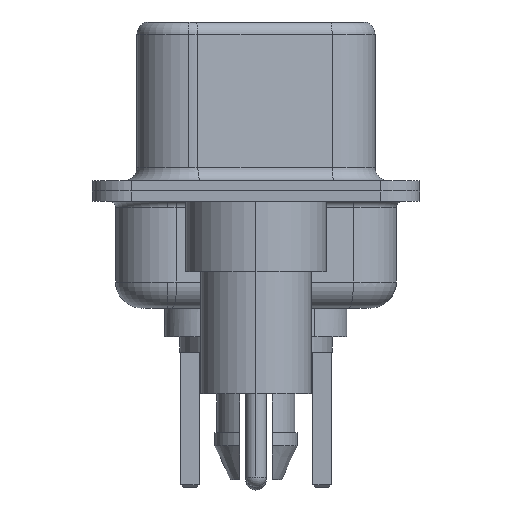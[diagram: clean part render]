
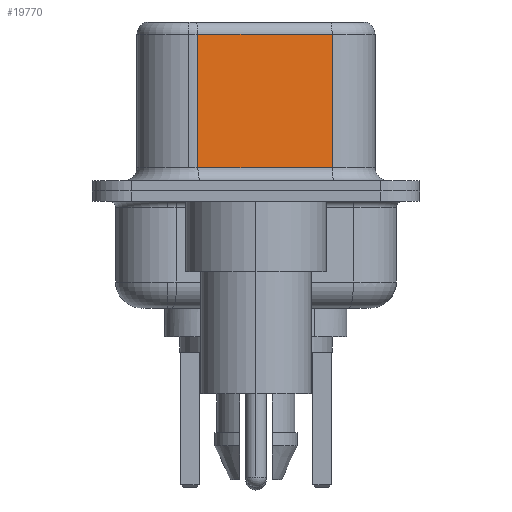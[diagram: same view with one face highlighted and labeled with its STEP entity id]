
A CAD part, left-side view. The second image highlights one B-rep face of the part: STEP entity #19770.
In plain terms, the highlighted planar face has unit normal (-0.985, -0.174, 0).
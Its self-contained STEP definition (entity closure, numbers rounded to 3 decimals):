
#413 = DIRECTION ( 'NONE',  ( -0.174, 0.985, 0. ) ) ;
#550 = LINE ( 'NONE', #19320, #12121 ) ;
#958 = EDGE_LOOP ( 'NONE', ( #11411, #16960, #17148, #9947 ) ) ;
#2748 = CARTESIAN_POINT ( 'NONE',  ( 4.565, -2.927, 6.02 ) ) ;
#3554 = EDGE_CURVE ( 'NONE', #14874, #12999, #9833, .T. ) ;
#4415 = PLANE ( 'NONE',  #17181 ) ;
#4439 = LINE ( 'NONE', #18417, #16595 ) ;
#6011 = DIRECTION ( 'NONE',  ( -0.174, 0.985, 0. ) ) ;
#6366 = FACE_OUTER_BOUND ( 'NONE', #958, .T. ) ;
#6947 = VECTOR ( 'NONE', #7154, 1000. ) ;
#7154 = DIRECTION ( 'NONE',  ( 0., 0., -1. ) ) ;
#7418 = CARTESIAN_POINT ( 'NONE',  ( 3.655, 2.233, 0.9 ) ) ;
#8909 = DIRECTION ( 'NONE',  ( 0., 0., -1. ) ) ;
#9833 = LINE ( 'NONE', #11067, #17757 ) ;
#9947 = ORIENTED_EDGE ( 'NONE', *, *, #3554, .T. ) ;
#10790 = CARTESIAN_POINT ( 'NONE',  ( 3.655, 2.233, 6.02 ) ) ;
#11067 = CARTESIAN_POINT ( 'NONE',  ( 4.565, -2.927, 0.9 ) ) ;
#11411 = ORIENTED_EDGE ( 'NONE', *, *, #14784, .F. ) ;
#11913 = CARTESIAN_POINT ( 'NONE',  ( 4.565, -2.927, 6.52 ) ) ;
#12121 = VECTOR ( 'NONE', #413, 1000. ) ;
#12999 = VERTEX_POINT ( 'NONE', #16021 ) ;
#13136 = DIRECTION ( 'NONE',  ( 0.174, -0.985, 0. ) ) ;
#14784 = EDGE_CURVE ( 'NONE', #19141, #12999, #14883, .T. ) ;
#14874 = VERTEX_POINT ( 'NONE', #7418 ) ;
#14883 = LINE ( 'NONE', #11913, #6947 ) ;
#15201 = EDGE_CURVE ( 'NONE', #19141, #16114, #550, .T. ) ;
#15424 = CARTESIAN_POINT ( 'NONE',  ( 4.565, -2.927, 6.52 ) ) ;
#15483 = EDGE_CURVE ( 'NONE', #16114, #14874, #4439, .T. ) ;
#15486 = DIRECTION ( 'NONE',  ( 0.985, 0.174, 0. ) ) ;
#16021 = CARTESIAN_POINT ( 'NONE',  ( 4.565, -2.927, 0.9 ) ) ;
#16114 = VERTEX_POINT ( 'NONE', #10790 ) ;
#16595 = VECTOR ( 'NONE', #8909, 1000. ) ;
#16960 = ORIENTED_EDGE ( 'NONE', *, *, #15201, .T. ) ;
#17148 = ORIENTED_EDGE ( 'NONE', *, *, #15483, .T. ) ;
#17181 = AXIS2_PLACEMENT_3D ( 'NONE', #15424, #15486, #6011 ) ;
#17757 = VECTOR ( 'NONE', #13136, 1000. ) ;
#18417 = CARTESIAN_POINT ( 'NONE',  ( 3.655, 2.233, 6.52 ) ) ;
#19141 = VERTEX_POINT ( 'NONE', #2748 ) ;
#19320 = CARTESIAN_POINT ( 'NONE',  ( 4.565, -2.927, 6.02 ) ) ;
#19770 = ADVANCED_FACE ( 'NONE', ( #6366 ), #4415, .F. ) ;
